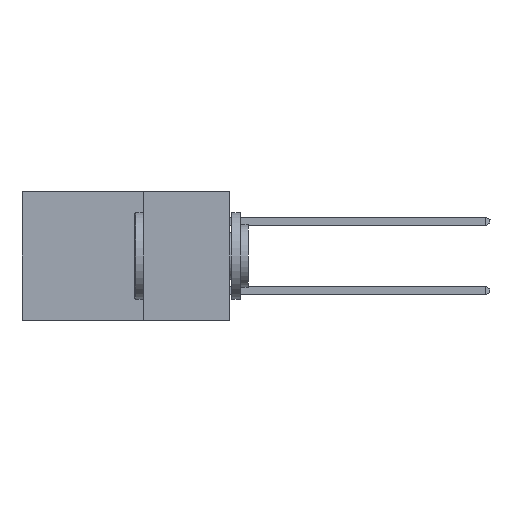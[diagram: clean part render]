
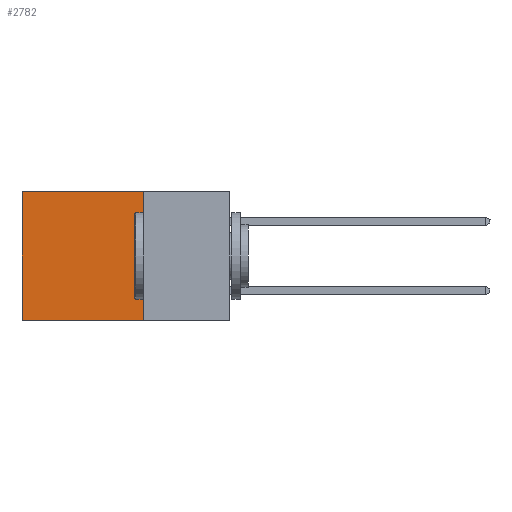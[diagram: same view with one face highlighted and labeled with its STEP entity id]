
A CAD part, left-side view. The second image highlights one B-rep face of the part: STEP entity #2782.
In plain terms, the highlighted planar face has unit normal (-1, 0, 0).
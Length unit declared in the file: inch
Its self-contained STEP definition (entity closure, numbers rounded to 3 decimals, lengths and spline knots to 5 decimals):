
#404 = CARTESIAN_POINT ( 'NONE',  ( 0.298, 0.25, 0. ) ) ;
#483 = DIRECTION ( 'NONE',  ( 0., 1., 0. ) ) ;
#612 = CARTESIAN_POINT ( 'NONE',  ( 0.298, 0.6, 0. ) ) ;
#804 = DIRECTION ( 'NONE',  ( 0., 0., -1. ) ) ;
#953 = LINE ( 'NONE', #404, #14396 ) ;
#1365 = ORIENTED_EDGE ( 'NONE', *, *, #17268, .F. ) ;
#2734 = CARTESIAN_POINT ( 'NONE',  ( 0.298, 0.6, 0. ) ) ;
#2782 = ADVANCED_FACE ( 'NONE', ( #3904 ), #5992, .F. ) ;
#2822 = CARTESIAN_POINT ( 'NONE',  ( 0.298, 0.25, 0. ) ) ;
#3904 = FACE_OUTER_BOUND ( 'NONE', #5744, .T. ) ;
#4156 = EDGE_CURVE ( 'NONE', #8170, #11786, #8452, .T. ) ;
#5744 = EDGE_LOOP ( 'NONE', ( #19032, #10100, #1365, #18274 ) ) ;
#5977 = LINE ( 'NONE', #17310, #8860 ) ;
#5992 = PLANE ( 'NONE',  #17643 ) ;
#6145 = CARTESIAN_POINT ( 'NONE',  ( 0.298, 0.25, 0. ) ) ;
#6390 = DIRECTION ( 'NONE',  ( 0., 0., -1. ) ) ;
#7054 = VECTOR ( 'NONE', #6390, 39.37008 ) ;
#8170 = VERTEX_POINT ( 'NONE', #11817 ) ;
#8396 = EDGE_CURVE ( 'NONE', #15302, #19552, #953, .T. ) ;
#8452 = LINE ( 'NONE', #18217, #13608 ) ;
#8860 = VECTOR ( 'NONE', #804, 39.37008 ) ;
#9121 = DIRECTION ( 'NONE',  ( 0., 1., 0. ) ) ;
#9797 = CARTESIAN_POINT ( 'NONE',  ( 0.298, 0.6, -0.37 ) ) ;
#10100 = ORIENTED_EDGE ( 'NONE', *, *, #4156, .F. ) ;
#11674 = DIRECTION ( 'NONE',  ( 0., 0., -1. ) ) ;
#11786 = VERTEX_POINT ( 'NONE', #9797 ) ;
#11817 = CARTESIAN_POINT ( 'NONE',  ( 0.298, 0.25, -0.37 ) ) ;
#12395 = EDGE_CURVE ( 'NONE', #19552, #11786, #13912, .T. ) ;
#13608 = VECTOR ( 'NONE', #9121, 39.37008 ) ;
#13912 = LINE ( 'NONE', #2734, #7054 ) ;
#14396 = VECTOR ( 'NONE', #483, 39.37008 ) ;
#15302 = VERTEX_POINT ( 'NONE', #2822 ) ;
#17268 = EDGE_CURVE ( 'NONE', #15302, #8170, #5977, .T. ) ;
#17310 = CARTESIAN_POINT ( 'NONE',  ( 0.298, 0.25, 0. ) ) ;
#17643 = AXIS2_PLACEMENT_3D ( 'NONE', #6145, #22462, #11674 ) ;
#18217 = CARTESIAN_POINT ( 'NONE',  ( 0.298, 0.25, -0.37 ) ) ;
#18274 = ORIENTED_EDGE ( 'NONE', *, *, #8396, .T. ) ;
#19032 = ORIENTED_EDGE ( 'NONE', *, *, #12395, .T. ) ;
#19552 = VERTEX_POINT ( 'NONE', #612 ) ;
#22462 = DIRECTION ( 'NONE',  ( 1., 0., 0. ) ) ;
